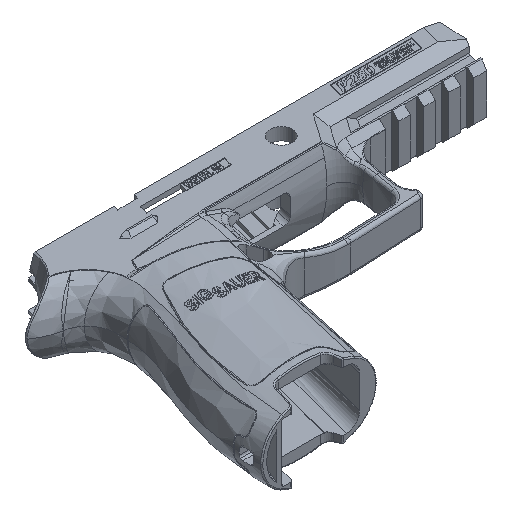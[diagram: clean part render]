
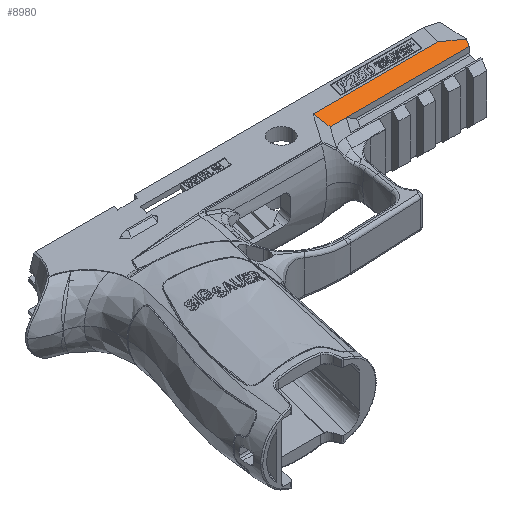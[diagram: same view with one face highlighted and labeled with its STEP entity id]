
A CAD part, isometric view. The second image highlights one B-rep face of the part: STEP entity #8980.
In plain terms, the highlighted planar face has unit normal (0, -0.602, 0.799).
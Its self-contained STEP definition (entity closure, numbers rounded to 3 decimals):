
#631 = VECTOR ( 'NONE', #13237, 1000. ) ;
#1173 = VECTOR ( 'NONE', #46927, 1000. ) ;
#2251 = LINE ( 'NONE', #50873, #631 ) ;
#4006 = CARTESIAN_POINT ( 'NONE',  ( 77.748, -20.312, 13.095 ) ) ;
#5303 = VECTOR ( 'NONE', #38509, 1000. ) ;
#5845 = ORIENTED_EDGE ( 'NONE', *, *, #31523, .T. ) ;
#8135 = EDGE_CURVE ( 'NONE', #21824, #31849, #29044, .T. ) ;
#8980 = ADVANCED_FACE ( 'NONE', ( #44617 ), #36557, .F. ) ;
#9223 = CARTESIAN_POINT ( 'NONE',  ( 82.229, -23.787, 10.477 ) ) ;
#9368 = VERTEX_POINT ( 'NONE', #55722 ) ;
#9522 = DIRECTION ( 'NONE',  ( -0.935, 0.283, 0.214 ) ) ;
#10405 = DIRECTION ( 'NONE',  ( 0., -0.799, -0.602 ) ) ;
#10686 = LINE ( 'NONE', #4006, #36961 ) ;
#11152 = VERTEX_POINT ( 'NONE', #27072 ) ;
#13237 = DIRECTION ( 'NONE',  ( 0.384, -0.737, -0.556 ) ) ;
#13826 = CARTESIAN_POINT ( 'NONE',  ( 82.263, -23.66, 10.573 ) ) ;
#15022 = ORIENTED_EDGE ( 'NONE', *, *, #8135, .F. ) ;
#15482 = CARTESIAN_POINT ( 'NONE',  ( 82.753, -23.66, 10.573 ) ) ;
#16869 = CARTESIAN_POINT ( 'NONE',  ( 32.876, -23.66, 10.573 ) ) ;
#20911 = DIRECTION ( 'NONE',  ( 1., 0., 0. ) ) ;
#21824 = VERTEX_POINT ( 'NONE', #16869 ) ;
#22279 = CARTESIAN_POINT ( 'NONE',  ( 82.753, -23.66, 10.573 ) ) ;
#22568 = EDGE_CURVE ( 'NONE', #66198, #31849, #2251, .T. ) ;
#26029 = CARTESIAN_POINT ( 'NONE',  ( 82.753, -19.199, 13.934 ) ) ;
#27072 = CARTESIAN_POINT ( 'NONE',  ( 82.753, -21.829, 11.952 ) ) ;
#27716 = EDGE_CURVE ( 'NONE', #58710, #21824, #33220, .T. ) ;
#28199 = LINE ( 'NONE', #9223, #40484 ) ;
#29044 = LINE ( 'NONE', #15482, #1173 ) ;
#31523 = EDGE_CURVE ( 'NONE', #58710, #11152, #28199, .T. ) ;
#31849 = VERTEX_POINT ( 'NONE', #48886 ) ;
#32556 = ORIENTED_EDGE ( 'NONE', *, *, #48303, .F. ) ;
#33220 = LINE ( 'NONE', #22279, #5303 ) ;
#36019 = EDGE_CURVE ( 'NONE', #11152, #9368, #10686, .T. ) ;
#36557 = PLANE ( 'NONE',  #66054 ) ;
#36961 = VECTOR ( 'NONE', #9522, 1000. ) ;
#38509 = DIRECTION ( 'NONE',  ( -1., 0., 0. ) ) ;
#40484 = VECTOR ( 'NONE', #61726, 1000. ) ;
#41765 = CARTESIAN_POINT ( 'NONE',  ( 37.5, -19.199, 13.934 ) ) ;
#41866 = DIRECTION ( 'NONE',  ( 0., 0.602, -0.799 ) ) ;
#42456 = ORIENTED_EDGE ( 'NONE', *, *, #22568, .T. ) ;
#44038 = ORIENTED_EDGE ( 'NONE', *, *, #36019, .T. ) ;
#44617 = FACE_OUTER_BOUND ( 'NONE', #45345, .T. ) ;
#45345 = EDGE_LOOP ( 'NONE', ( #5845, #44038, #32556, #42456, #15022, #62494 ) ) ;
#46927 = DIRECTION ( 'NONE',  ( -1., 0., 0. ) ) ;
#48303 = EDGE_CURVE ( 'NONE', #66198, #9368, #64244, .T. ) ;
#48886 = CARTESIAN_POINT ( 'NONE',  ( 26.436, -23.66, 10.573 ) ) ;
#50873 = CARTESIAN_POINT ( 'NONE',  ( 29.937, -30.385, 5.505 ) ) ;
#51956 = VECTOR ( 'NONE', #20911, 1000. ) ;
#55722 = CARTESIAN_POINT ( 'NONE',  ( 74.078, -19.199, 13.934 ) ) ;
#58710 = VERTEX_POINT ( 'NONE', #13826 ) ;
#61726 = DIRECTION ( 'NONE',  ( 0.209, 0.781, 0.588 ) ) ;
#62122 = CARTESIAN_POINT ( 'NONE',  ( 24.114, -19.199, 13.934 ) ) ;
#62494 = ORIENTED_EDGE ( 'NONE', *, *, #27716, .F. ) ;
#64244 = LINE ( 'NONE', #41765, #51956 ) ;
#66054 = AXIS2_PLACEMENT_3D ( 'NONE', #26029, #41866, #10405 ) ;
#66198 = VERTEX_POINT ( 'NONE', #62122 ) ;
